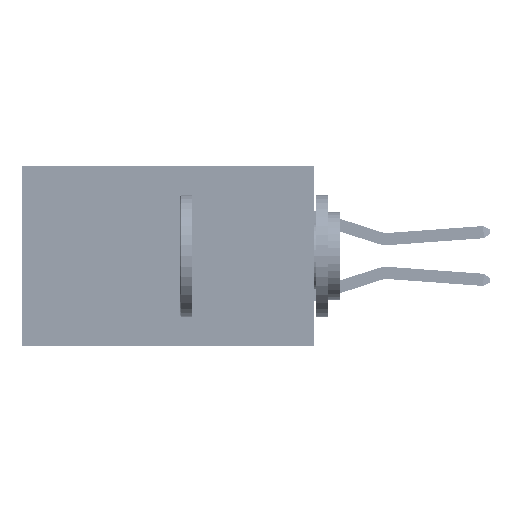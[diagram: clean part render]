
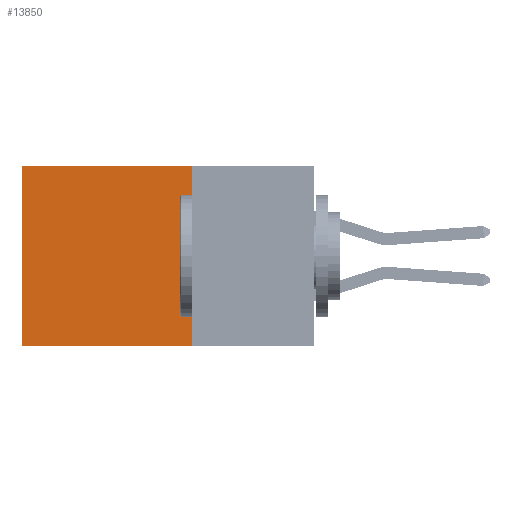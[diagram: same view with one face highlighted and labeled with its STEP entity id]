
A CAD part, left-side view. The second image highlights one B-rep face of the part: STEP entity #13850.
In plain terms, the highlighted planar face has unit normal (-1, 0, 0).
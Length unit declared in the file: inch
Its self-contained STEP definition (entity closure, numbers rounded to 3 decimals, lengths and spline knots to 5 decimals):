
#2175 = CARTESIAN_POINT ( 'NONE',  ( 0.2875, 0.25, 0. ) ) ;
#2256 = CARTESIAN_POINT ( 'NONE',  ( 0.2875, 0.25, 0. ) ) ;
#2347 = VECTOR ( 'NONE', #7173, 39.37008 ) ;
#2585 = LINE ( 'NONE', #45350, #39860 ) ;
#4874 = VECTOR ( 'NONE', #34211, 39.37008 ) ;
#5349 = EDGE_LOOP ( 'NONE', ( #22439, #40659, #17003, #37803 ) ) ;
#5778 = DIRECTION ( 'NONE',  ( 0., 1., 0. ) ) ;
#7173 = DIRECTION ( 'NONE',  ( 0., 0., -1. ) ) ;
#11577 = DIRECTION ( 'NONE',  ( 0., 0., -1. ) ) ;
#12904 = VERTEX_POINT ( 'NONE', #2256 ) ;
#13140 = CARTESIAN_POINT ( 'NONE',  ( 0.2875, 0.25, -0.37 ) ) ;
#13850 = ADVANCED_FACE ( 'NONE', ( #40875 ), #36417, .F. ) ;
#14188 = VERTEX_POINT ( 'NONE', #13140 ) ;
#14630 = CARTESIAN_POINT ( 'NONE',  ( 0.2875, 0.25, 0. ) ) ;
#16473 = LINE ( 'NONE', #32792, #2347 ) ;
#17003 = ORIENTED_EDGE ( 'NONE', *, *, #19257, .F. ) ;
#17037 = AXIS2_PLACEMENT_3D ( 'NONE', #14630, #18416, #11577 ) ;
#17500 = VERTEX_POINT ( 'NONE', #23794 ) ;
#18416 = DIRECTION ( 'NONE',  ( 1., 0., 0. ) ) ;
#19257 = EDGE_CURVE ( 'NONE', #12904, #14188, #2585, .T. ) ;
#19988 = CARTESIAN_POINT ( 'NONE',  ( 0.2875, 0.25, -0.37 ) ) ;
#22439 = ORIENTED_EDGE ( 'NONE', *, *, #44919, .T. ) ;
#23794 = CARTESIAN_POINT ( 'NONE',  ( 0.2875, 0.6, -0.37 ) ) ;
#26863 = EDGE_CURVE ( 'NONE', #12904, #45052, #39611, .T. ) ;
#29762 = CARTESIAN_POINT ( 'NONE',  ( 0.2875, 0.6, 0. ) ) ;
#30863 = DIRECTION ( 'NONE',  ( 0., 0., -1. ) ) ;
#31454 = LINE ( 'NONE', #19988, #4874 ) ;
#32792 = CARTESIAN_POINT ( 'NONE',  ( 0.2875, 0.6, 0. ) ) ;
#34211 = DIRECTION ( 'NONE',  ( 0., 1., 0. ) ) ;
#36417 = PLANE ( 'NONE',  #17037 ) ;
#37803 = ORIENTED_EDGE ( 'NONE', *, *, #26863, .T. ) ;
#39611 = LINE ( 'NONE', #2175, #46352 ) ;
#39860 = VECTOR ( 'NONE', #30863, 39.37008 ) ;
#40659 = ORIENTED_EDGE ( 'NONE', *, *, #42287, .F. ) ;
#40875 = FACE_OUTER_BOUND ( 'NONE', #5349, .T. ) ;
#42287 = EDGE_CURVE ( 'NONE', #14188, #17500, #31454, .T. ) ;
#44919 = EDGE_CURVE ( 'NONE', #45052, #17500, #16473, .T. ) ;
#45052 = VERTEX_POINT ( 'NONE', #29762 ) ;
#45350 = CARTESIAN_POINT ( 'NONE',  ( 0.2875, 0.25, 0. ) ) ;
#46352 = VECTOR ( 'NONE', #5778, 39.37008 ) ;
